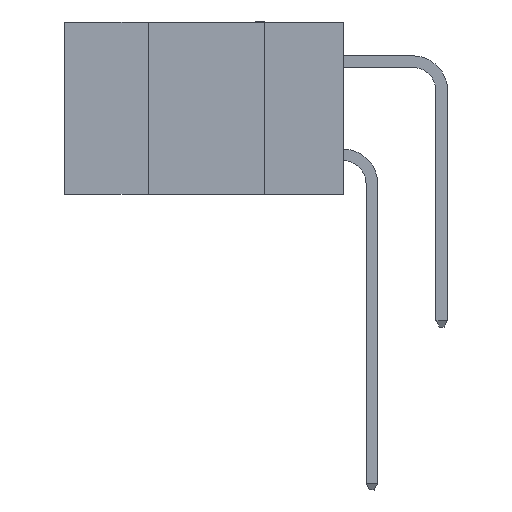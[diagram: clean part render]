
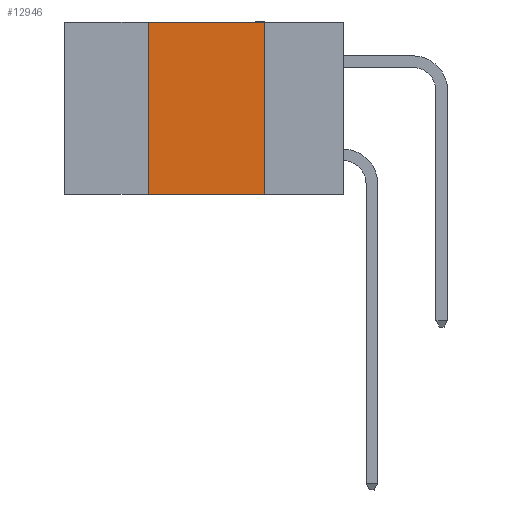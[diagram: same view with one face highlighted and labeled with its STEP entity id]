
A CAD part, left-side view. The second image highlights one B-rep face of the part: STEP entity #12946.
In plain terms, the highlighted planar face has unit normal (-1, 0, 0).
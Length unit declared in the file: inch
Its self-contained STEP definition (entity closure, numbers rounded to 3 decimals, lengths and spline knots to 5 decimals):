
#947 = LINE ( 'NONE', #22950, #21140 ) ;
#965 = DIRECTION ( 'NONE',  ( 0., 0., -1. ) ) ;
#1464 = CARTESIAN_POINT ( 'NONE',  ( 0., 0.42, 0. ) ) ;
#1964 = EDGE_CURVE ( 'NONE', #9080, #18795, #13175, .T. ) ;
#2899 = PLANE ( 'NONE',  #15229 ) ;
#4956 = VECTOR ( 'NONE', #17976, 39.37008 ) ;
#6027 = EDGE_CURVE ( 'NONE', #9080, #12166, #947, .T. ) ;
#7579 = CARTESIAN_POINT ( 'NONE',  ( 0., 0.17, 0. ) ) ;
#7613 = DIRECTION ( 'NONE',  ( 1., 0., 0. ) ) ;
#7914 = ORIENTED_EDGE ( 'NONE', *, *, #24387, .F. ) ;
#9080 = VERTEX_POINT ( 'NONE', #11346 ) ;
#9746 = ORIENTED_EDGE ( 'NONE', *, *, #1964, .T. ) ;
#10651 = DIRECTION ( 'NONE',  ( 0., 0., 1. ) ) ;
#11346 = CARTESIAN_POINT ( 'NONE',  ( 0., 0.42, -0.37 ) ) ;
#11442 = LINE ( 'NONE', #23557, #21839 ) ;
#12166 = VERTEX_POINT ( 'NONE', #1464 ) ;
#12184 = FACE_OUTER_BOUND ( 'NONE', #23757, .T. ) ;
#12617 = VECTOR ( 'NONE', #25543, 39.37008 ) ;
#12946 = ADVANCED_FACE ( 'NONE', ( #12184 ), #2899, .F. ) ;
#13175 = LINE ( 'NONE', #15705, #4956 ) ;
#15229 = AXIS2_PLACEMENT_3D ( 'NONE', #23187, #7613, #965 ) ;
#15461 = DIRECTION ( 'NONE',  ( 0., -1., 0. ) ) ;
#15705 = CARTESIAN_POINT ( 'NONE',  ( 0., 0.6, -0.37 ) ) ;
#16358 = LINE ( 'NONE', #17440, #12617 ) ;
#17440 = CARTESIAN_POINT ( 'NONE',  ( 0., 0.17, 0. ) ) ;
#17513 = ORIENTED_EDGE ( 'NONE', *, *, #22074, .F. ) ;
#17976 = DIRECTION ( 'NONE',  ( 0., -1., 0. ) ) ;
#18795 = VERTEX_POINT ( 'NONE', #24921 ) ;
#21140 = VECTOR ( 'NONE', #10651, 39.37008 ) ;
#21839 = VECTOR ( 'NONE', #15461, 39.37008 ) ;
#22074 = EDGE_CURVE ( 'NONE', #12166, #25024, #11442, .T. ) ;
#22950 = CARTESIAN_POINT ( 'NONE',  ( 0., 0.42, 0. ) ) ;
#23187 = CARTESIAN_POINT ( 'NONE',  ( 0., 0.6, 0. ) ) ;
#23557 = CARTESIAN_POINT ( 'NONE',  ( 0., 0.6, 0. ) ) ;
#23757 = EDGE_LOOP ( 'NONE', ( #7914, #17513, #25914, #9746 ) ) ;
#24387 = EDGE_CURVE ( 'NONE', #25024, #18795, #16358, .T. ) ;
#24921 = CARTESIAN_POINT ( 'NONE',  ( 0., 0.17, -0.37 ) ) ;
#25024 = VERTEX_POINT ( 'NONE', #7579 ) ;
#25543 = DIRECTION ( 'NONE',  ( 0., 0., -1. ) ) ;
#25914 = ORIENTED_EDGE ( 'NONE', *, *, #6027, .F. ) ;
